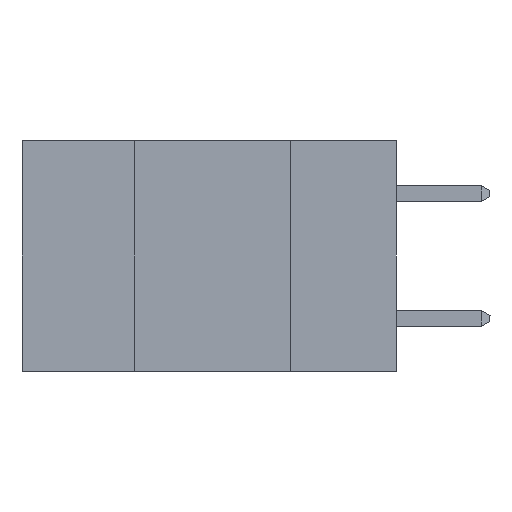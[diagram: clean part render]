
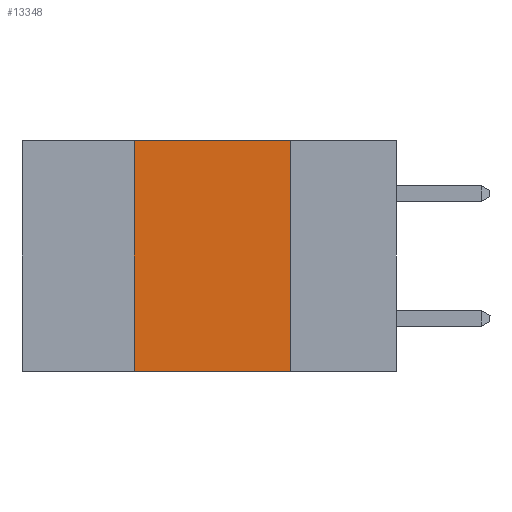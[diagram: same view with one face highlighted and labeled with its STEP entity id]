
A CAD part, left-side view. The second image highlights one B-rep face of the part: STEP entity #13348.
In plain terms, the highlighted planar face has unit normal (-1, 0, 0).
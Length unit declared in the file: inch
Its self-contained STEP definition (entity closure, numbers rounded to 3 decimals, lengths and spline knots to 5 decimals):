
#134 = LINE ( 'NONE', #13997, #15716 ) ;
#899 = EDGE_CURVE ( 'NONE', #16984, #11504, #9664, .T. ) ;
#995 = FACE_OUTER_BOUND ( 'NONE', #7488, .T. ) ;
#1488 = VECTOR ( 'NONE', #18736, 39.37008 ) ;
#2152 = LINE ( 'NONE', #9016, #16772 ) ;
#2527 = CARTESIAN_POINT ( 'NONE',  ( 0., 0.17, 0. ) ) ;
#3356 = EDGE_CURVE ( 'NONE', #16049, #11504, #134, .T. ) ;
#3647 = DIRECTION ( 'NONE',  ( 0., 0., -1. ) ) ;
#3742 = ORIENTED_EDGE ( 'NONE', *, *, #14478, .F. ) ;
#4052 = AXIS2_PLACEMENT_3D ( 'NONE', #9629, #12669, #3647 ) ;
#5104 = PLANE ( 'NONE',  #4052 ) ;
#5172 = ORIENTED_EDGE ( 'NONE', *, *, #3356, .T. ) ;
#5681 = VECTOR ( 'NONE', #11783, 39.37008 ) ;
#5811 = EDGE_CURVE ( 'NONE', #16049, #10201, #13542, .T. ) ;
#5879 = CARTESIAN_POINT ( 'NONE',  ( 0., 0.42, 0. ) ) ;
#7488 = EDGE_LOOP ( 'NONE', ( #18801, #3742, #12254, #5172 ) ) ;
#9016 = CARTESIAN_POINT ( 'NONE',  ( 0., 0.6, 0. ) ) ;
#9629 = CARTESIAN_POINT ( 'NONE',  ( 0., 0.6, 0. ) ) ;
#9664 = LINE ( 'NONE', #12555, #5681 ) ;
#10201 = VERTEX_POINT ( 'NONE', #5879 ) ;
#10522 = DIRECTION ( 'NONE',  ( 0., -1., 0. ) ) ;
#11152 = CARTESIAN_POINT ( 'NONE',  ( 0., 0.42, -0.37 ) ) ;
#11504 = VERTEX_POINT ( 'NONE', #12781 ) ;
#11783 = DIRECTION ( 'NONE',  ( 0., 0., -1. ) ) ;
#12254 = ORIENTED_EDGE ( 'NONE', *, *, #5811, .F. ) ;
#12555 = CARTESIAN_POINT ( 'NONE',  ( 0., 0.17, -0.37 ) ) ;
#12669 = DIRECTION ( 'NONE',  ( 1., 0., 0. ) ) ;
#12781 = CARTESIAN_POINT ( 'NONE',  ( 0., 0.17, -0.37 ) ) ;
#13348 = ADVANCED_FACE ( 'NONE', ( #995 ), #5104, .F. ) ;
#13542 = LINE ( 'NONE', #19455, #1488 ) ;
#13973 = DIRECTION ( 'NONE',  ( 0., -1., 0. ) ) ;
#13997 = CARTESIAN_POINT ( 'NONE',  ( 0., 0.6, -0.37 ) ) ;
#14478 = EDGE_CURVE ( 'NONE', #10201, #16984, #2152, .T. ) ;
#15716 = VECTOR ( 'NONE', #13973, 39.37008 ) ;
#16049 = VERTEX_POINT ( 'NONE', #11152 ) ;
#16772 = VECTOR ( 'NONE', #10522, 39.37008 ) ;
#16984 = VERTEX_POINT ( 'NONE', #2527 ) ;
#18736 = DIRECTION ( 'NONE',  ( 0., 0., 1. ) ) ;
#18801 = ORIENTED_EDGE ( 'NONE', *, *, #899, .F. ) ;
#19455 = CARTESIAN_POINT ( 'NONE',  ( 0., 0.42, -0.37 ) ) ;
